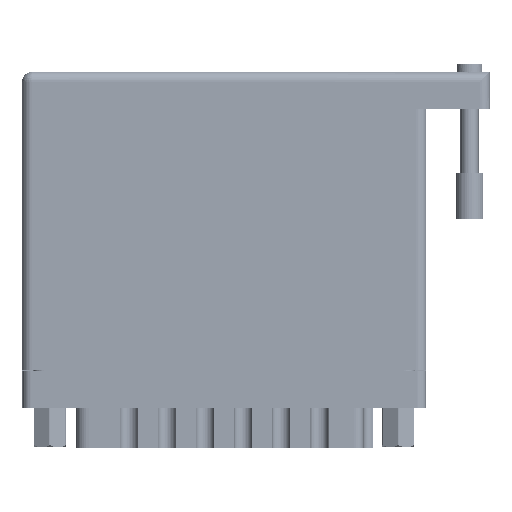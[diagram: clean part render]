
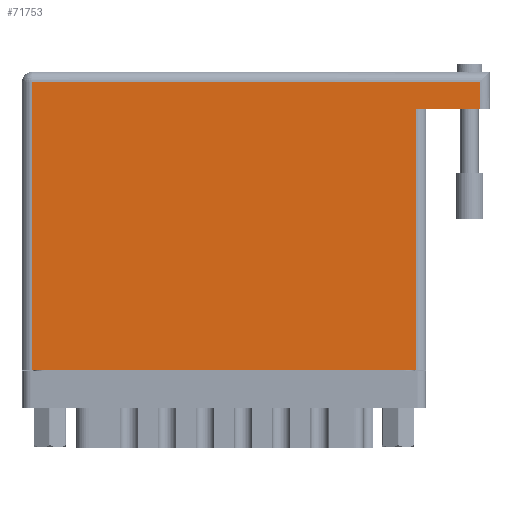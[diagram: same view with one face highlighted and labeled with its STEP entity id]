
A CAD part, front view. The second image highlights one B-rep face of the part: STEP entity #71753.
In plain terms, the highlighted face is planar.
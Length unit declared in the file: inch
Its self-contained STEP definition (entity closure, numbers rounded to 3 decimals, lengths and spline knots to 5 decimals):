
#3379 = PLANE ( 'NONE',  #26850 ) ;
#4851 = LINE ( 'NONE', #12588, #62419 ) ;
#5820 = DIRECTION ( 'NONE',  ( 1., 0., 0. ) ) ;
#5858 = ORIENTED_EDGE ( 'NONE', *, *, #96451, .T. ) ;
#11608 = DIRECTION ( 'NONE',  ( -1., 0., 0. ) ) ;
#12089 = CARTESIAN_POINT ( 'NONE',  ( 2.685, 0., 0. ) ) ;
#12588 = CARTESIAN_POINT ( 'NONE',  ( 3.19, 1.774, 0. ) ) ;
#15583 = ORIENTED_EDGE ( 'NONE', *, *, #74289, .T. ) ;
#15687 = CARTESIAN_POINT ( 'NONE',  ( 2.685, 1.774, 0. ) ) ;
#19876 = CARTESIAN_POINT ( 'NONE',  ( 0.07, 1.96, 0. ) ) ;
#20009 = LINE ( 'NONE', #21975, #58335 ) ;
#20513 = DIRECTION ( 'NONE',  ( 0., -1., 0. ) ) ;
#21975 = CARTESIAN_POINT ( 'NONE',  ( 0., 0., 0. ) ) ;
#22852 = VECTOR ( 'NONE', #20513, 39.37008 ) ;
#25978 = VERTEX_POINT ( 'NONE', #62977 ) ;
#26850 = AXIS2_PLACEMENT_3D ( 'NONE', #36298, #93764, #11608 ) ;
#27746 = FACE_OUTER_BOUND ( 'NONE', #104291, .T. ) ;
#28025 = DIRECTION ( 'NONE',  ( -1., 0., 0. ) ) ;
#29185 = LINE ( 'NONE', #45494, #22852 ) ;
#32547 = EDGE_CURVE ( 'NONE', #78955, #25978, #29185, .T. ) ;
#34471 = CARTESIAN_POINT ( 'NONE',  ( 2.685, 1.774, 0. ) ) ;
#35921 = VERTEX_POINT ( 'NONE', #12089 ) ;
#36298 = CARTESIAN_POINT ( 'NONE',  ( 0., 2.03, 0. ) ) ;
#38047 = DIRECTION ( 'NONE',  ( 0., 1., 0. ) ) ;
#42489 = LINE ( 'NONE', #15687, #74487 ) ;
#43526 = VERTEX_POINT ( 'NONE', #34471 ) ;
#44943 = LINE ( 'NONE', #55522, #94753 ) ;
#45494 = CARTESIAN_POINT ( 'NONE',  ( 0.07, 0., 0. ) ) ;
#51194 = VERTEX_POINT ( 'NONE', #103402 ) ;
#53292 = VECTOR ( 'NONE', #66069, 39.37008 ) ;
#55522 = CARTESIAN_POINT ( 'NONE',  ( 3.12, 2.03, 0. ) ) ;
#57460 = EDGE_CURVE ( 'NONE', #51194, #43526, #4851, .T. ) ;
#58335 = VECTOR ( 'NONE', #5820, 39.37008 ) ;
#60791 = ORIENTED_EDGE ( 'NONE', *, *, #75257, .T. ) ;
#62419 = VECTOR ( 'NONE', #28025, 39.37008 ) ;
#62977 = CARTESIAN_POINT ( 'NONE',  ( 0.07, 0., 0. ) ) ;
#66069 = DIRECTION ( 'NONE',  ( -1., 0., 0. ) ) ;
#71753 = ADVANCED_FACE ( 'NONE', ( #27746 ), #3379, .F. ) ;
#74289 = EDGE_CURVE ( 'NONE', #35921, #43526, #42489, .T. ) ;
#74487 = VECTOR ( 'NONE', #105009, 39.37008 ) ;
#75257 = EDGE_CURVE ( 'NONE', #51194, #85025, #44943, .T. ) ;
#75662 = CARTESIAN_POINT ( 'NONE',  ( 0., 1.96, 0. ) ) ;
#76852 = CARTESIAN_POINT ( 'NONE',  ( 3.12, 1.96, 0. ) ) ;
#78955 = VERTEX_POINT ( 'NONE', #19876 ) ;
#82178 = ORIENTED_EDGE ( 'NONE', *, *, #57460, .F. ) ;
#82352 = EDGE_CURVE ( 'NONE', #25978, #35921, #20009, .T. ) ;
#85025 = VERTEX_POINT ( 'NONE', #76852 ) ;
#86735 = ORIENTED_EDGE ( 'NONE', *, *, #32547, .T. ) ;
#93764 = DIRECTION ( 'NONE',  ( 0., 0., -1. ) ) ;
#94753 = VECTOR ( 'NONE', #38047, 39.37008 ) ;
#96451 = EDGE_CURVE ( 'NONE', #85025, #78955, #96698, .T. ) ;
#96698 = LINE ( 'NONE', #75662, #53292 ) ;
#102817 = ORIENTED_EDGE ( 'NONE', *, *, #82352, .T. ) ;
#103402 = CARTESIAN_POINT ( 'NONE',  ( 3.12, 1.774, 0. ) ) ;
#104291 = EDGE_LOOP ( 'NONE', ( #102817, #15583, #82178, #60791, #5858, #86735 ) ) ;
#105009 = DIRECTION ( 'NONE',  ( 0., 1., 0. ) ) ;
